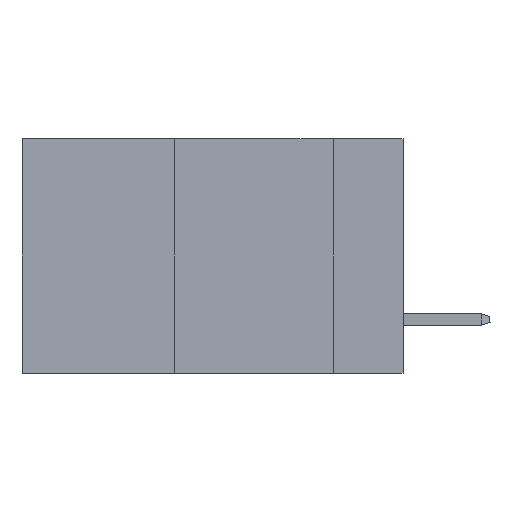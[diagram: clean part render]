
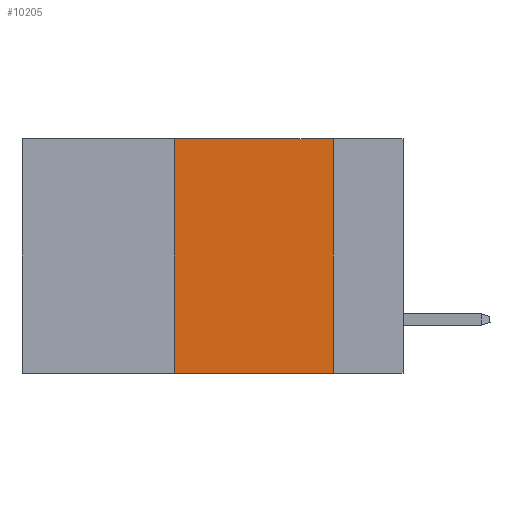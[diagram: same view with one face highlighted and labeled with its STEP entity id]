
A CAD part, left-side view. The second image highlights one B-rep face of the part: STEP entity #10205.
In plain terms, the highlighted planar face has unit normal (-1, 0, 0).
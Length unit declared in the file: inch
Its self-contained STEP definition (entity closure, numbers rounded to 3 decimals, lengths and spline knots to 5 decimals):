
#60 = DIRECTION ( 'NONE',  ( 0., 0., 1. ) ) ;
#171 = VECTOR ( 'NONE', #3643, 39.37008 ) ;
#430 = EDGE_CURVE ( 'NONE', #3433, #8158, #2319, .T. ) ;
#505 = DIRECTION ( 'NONE',  ( 0., -1., 0. ) ) ;
#775 = EDGE_LOOP ( 'NONE', ( #14778, #9904, #11494, #15788 ) ) ;
#1339 = VECTOR ( 'NONE', #505, 39.37008 ) ;
#1771 = CARTESIAN_POINT ( 'NONE',  ( 0., 0.6, 0. ) ) ;
#2319 = LINE ( 'NONE', #3736, #171 ) ;
#2468 = VECTOR ( 'NONE', #60, 39.37008 ) ;
#3177 = CARTESIAN_POINT ( 'NONE',  ( 0., 0.36, 0. ) ) ;
#3433 = VERTEX_POINT ( 'NONE', #6570 ) ;
#3643 = DIRECTION ( 'NONE',  ( 0., 0., -1. ) ) ;
#3736 = CARTESIAN_POINT ( 'NONE',  ( 0., 0.11, 0. ) ) ;
#5026 = VERTEX_POINT ( 'NONE', #5574 ) ;
#5574 = CARTESIAN_POINT ( 'NONE',  ( 0., 0.36, -0.37 ) ) ;
#5777 = LINE ( 'NONE', #12697, #1339 ) ;
#6570 = CARTESIAN_POINT ( 'NONE',  ( 0., 0.11, 0. ) ) ;
#7209 = EDGE_CURVE ( 'NONE', #11124, #3433, #13055, .T. ) ;
#7356 = EDGE_CURVE ( 'NONE', #5026, #11124, #16276, .T. ) ;
#8158 = VERTEX_POINT ( 'NONE', #10528 ) ;
#8542 = AXIS2_PLACEMENT_3D ( 'NONE', #1771, #15134, #12623 ) ;
#8894 = EDGE_CURVE ( 'NONE', #5026, #8158, #5777, .T. ) ;
#9904 = ORIENTED_EDGE ( 'NONE', *, *, #7209, .F. ) ;
#10205 = ADVANCED_FACE ( 'NONE', ( #13986 ), #15303, .F. ) ;
#10528 = CARTESIAN_POINT ( 'NONE',  ( 0., 0.11, -0.37 ) ) ;
#11124 = VERTEX_POINT ( 'NONE', #3177 ) ;
#11494 = ORIENTED_EDGE ( 'NONE', *, *, #7356, .F. ) ;
#11735 = DIRECTION ( 'NONE',  ( 0., -1., 0. ) ) ;
#12236 = CARTESIAN_POINT ( 'NONE',  ( 0., 0.36, 0. ) ) ;
#12620 = CARTESIAN_POINT ( 'NONE',  ( 0., 0.6, 0. ) ) ;
#12623 = DIRECTION ( 'NONE',  ( 0., 0., -1. ) ) ;
#12697 = CARTESIAN_POINT ( 'NONE',  ( 0., 0.6, -0.37 ) ) ;
#13055 = LINE ( 'NONE', #12620, #17588 ) ;
#13986 = FACE_OUTER_BOUND ( 'NONE', #775, .T. ) ;
#14778 = ORIENTED_EDGE ( 'NONE', *, *, #430, .F. ) ;
#15134 = DIRECTION ( 'NONE',  ( 1., 0., 0. ) ) ;
#15303 = PLANE ( 'NONE',  #8542 ) ;
#15788 = ORIENTED_EDGE ( 'NONE', *, *, #8894, .T. ) ;
#16276 = LINE ( 'NONE', #12236, #2468 ) ;
#17588 = VECTOR ( 'NONE', #11735, 39.37008 ) ;
